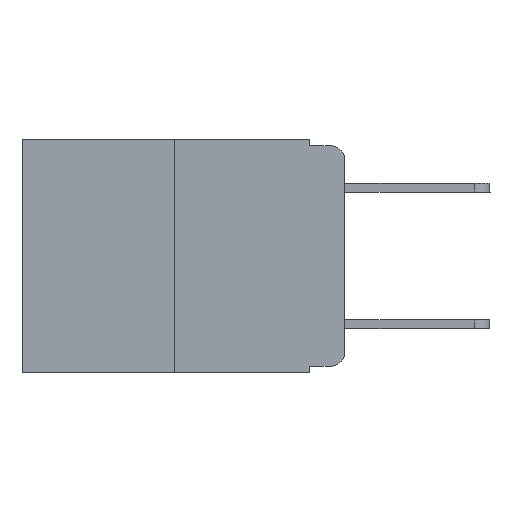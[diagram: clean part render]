
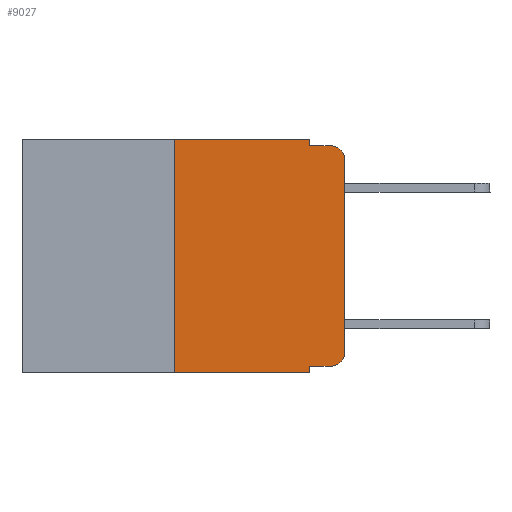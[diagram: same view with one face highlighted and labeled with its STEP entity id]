
A CAD part, left-side view. The second image highlights one B-rep face of the part: STEP entity #9027.
In plain terms, the highlighted planar face has unit normal (-1, 0, 0).
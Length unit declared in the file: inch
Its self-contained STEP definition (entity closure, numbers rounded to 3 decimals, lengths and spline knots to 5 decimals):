
#101 = LINE ( 'NONE', #2059, #4918 ) ;
#133 = LINE ( 'NONE', #5487, #2238 ) ;
#315 = DIRECTION ( 'NONE',  ( 0., -1., 0. ) ) ;
#328 = DIRECTION ( 'NONE',  ( 0., 0., -1. ) ) ;
#723 = CARTESIAN_POINT ( 'NONE',  ( 0., 0.051, -0.01 ) ) ;
#773 = CIRCLE ( 'NONE', #4574, 0.02 ) ;
#930 = ORIENTED_EDGE ( 'NONE', *, *, #2536, .F. ) ;
#1069 = AXIS2_PLACEMENT_3D ( 'NONE', #9760, #3588, #4391 ) ;
#1071 = EDGE_CURVE ( 'NONE', #6684, #6818, #6319, .T. ) ;
#1081 = CARTESIAN_POINT ( 'NONE',  ( 0., 0.473, 0. ) ) ;
#1154 = LINE ( 'NONE', #7395, #5694 ) ;
#1967 = DIRECTION ( 'NONE',  ( 0., 0., -1. ) ) ;
#2000 = EDGE_CURVE ( 'NONE', #10084, #7361, #8566, .T. ) ;
#2059 = CARTESIAN_POINT ( 'NONE',  ( 0., 0.051, 0. ) ) ;
#2163 = DIRECTION ( 'NONE',  ( -1., 0., 0. ) ) ;
#2238 = VECTOR ( 'NONE', #3946, 39.37008 ) ;
#2375 = CARTESIAN_POINT ( 'NONE',  ( 0., 0.051, -0.01 ) ) ;
#2395 = ORIENTED_EDGE ( 'NONE', *, *, #4846, .T. ) ;
#2536 = EDGE_CURVE ( 'NONE', #4348, #4883, #101, .T. ) ;
#2615 = AXIS2_PLACEMENT_3D ( 'NONE', #8414, #2163, #4628 ) ;
#2802 = DIRECTION ( 'NONE',  ( 0., -1., 0. ) ) ;
#2839 = CARTESIAN_POINT ( 'NONE',  ( 0., 0.051, -0.343 ) ) ;
#2976 = ORIENTED_EDGE ( 'NONE', *, *, #8283, .T. ) ;
#3493 = ORIENTED_EDGE ( 'NONE', *, *, #5857, .F. ) ;
#3586 = DIRECTION ( 'NONE',  ( 0., 0., 1. ) ) ;
#3588 = DIRECTION ( 'NONE',  ( 1., 0., 0. ) ) ;
#3708 = EDGE_CURVE ( 'NONE', #4954, #10084, #6498, .T. ) ;
#3941 = LINE ( 'NONE', #4165, #5410 ) ;
#3946 = DIRECTION ( 'NONE',  ( 0., 0., -1. ) ) ;
#4165 = CARTESIAN_POINT ( 'NONE',  ( 0., 0.051, -0.333 ) ) ;
#4207 = CARTESIAN_POINT ( 'NONE',  ( 0., 0.02, -0.333 ) ) ;
#4348 = VERTEX_POINT ( 'NONE', #9409 ) ;
#4374 = EDGE_CURVE ( 'NONE', #10076, #6104, #7677, .T. ) ;
#4391 = DIRECTION ( 'NONE',  ( 0., 0., -1. ) ) ;
#4407 = CARTESIAN_POINT ( 'NONE',  ( 0., 0.02, -0.313 ) ) ;
#4574 = AXIS2_PLACEMENT_3D ( 'NONE', #4407, #5123, #1967 ) ;
#4628 = DIRECTION ( 'NONE',  ( 0., 0., -1. ) ) ;
#4703 = CARTESIAN_POINT ( 'NONE',  ( 0., 0., 0. ) ) ;
#4775 = ORIENTED_EDGE ( 'NONE', *, *, #2000, .F. ) ;
#4846 = EDGE_CURVE ( 'NONE', #4954, #4883, #1154, .T. ) ;
#4883 = VERTEX_POINT ( 'NONE', #2839 ) ;
#4918 = VECTOR ( 'NONE', #328, 39.37008 ) ;
#4954 = VERTEX_POINT ( 'NONE', #8898 ) ;
#5003 = ORIENTED_EDGE ( 'NONE', *, *, #6383, .T. ) ;
#5123 = DIRECTION ( 'NONE',  ( -1., 0., 0. ) ) ;
#5276 = FACE_OUTER_BOUND ( 'NONE', #6933, .T. ) ;
#5410 = VECTOR ( 'NONE', #6280, 39.37008 ) ;
#5487 = CARTESIAN_POINT ( 'NONE',  ( 0., 0.051, 0. ) ) ;
#5499 = EDGE_CURVE ( 'NONE', #7713, #6684, #773, .T. ) ;
#5694 = VECTOR ( 'NONE', #2802, 39.37008 ) ;
#5857 = EDGE_CURVE ( 'NONE', #7361, #10076, #133, .T. ) ;
#6104 = VERTEX_POINT ( 'NONE', #9462 ) ;
#6280 = DIRECTION ( 'NONE',  ( 0., -1., 0. ) ) ;
#6319 = LINE ( 'NONE', #4703, #8135 ) ;
#6349 = DIRECTION ( 'NONE',  ( 0., -1., 0. ) ) ;
#6383 = EDGE_CURVE ( 'NONE', #6818, #6104, #9322, .T. ) ;
#6498 = LINE ( 'NONE', #7581, #7220 ) ;
#6684 = VERTEX_POINT ( 'NONE', #8740 ) ;
#6818 = VERTEX_POINT ( 'NONE', #8974 ) ;
#6933 = EDGE_LOOP ( 'NONE', ( #8978, #5003, #8326, #3493, #4775, #8273, #2395, #930, #2976, #9529 ) ) ;
#7220 = VECTOR ( 'NONE', #3586, 39.37008 ) ;
#7361 = VERTEX_POINT ( 'NONE', #8048 ) ;
#7395 = CARTESIAN_POINT ( 'NONE',  ( 0., 0.473, -0.343 ) ) ;
#7581 = CARTESIAN_POINT ( 'NONE',  ( 0., 0.25, 0. ) ) ;
#7677 = LINE ( 'NONE', #723, #8895 ) ;
#7713 = VERTEX_POINT ( 'NONE', #4207 ) ;
#8048 = CARTESIAN_POINT ( 'NONE',  ( 0., 0.051, 0. ) ) ;
#8135 = VECTOR ( 'NONE', #10170, 39.37008 ) ;
#8273 = ORIENTED_EDGE ( 'NONE', *, *, #3708, .F. ) ;
#8283 = EDGE_CURVE ( 'NONE', #4348, #7713, #3941, .T. ) ;
#8326 = ORIENTED_EDGE ( 'NONE', *, *, #4374, .F. ) ;
#8414 = CARTESIAN_POINT ( 'NONE',  ( 0., 0.02, -0.03 ) ) ;
#8566 = LINE ( 'NONE', #1081, #10172 ) ;
#8719 = CARTESIAN_POINT ( 'NONE',  ( 0., 0.25, 0. ) ) ;
#8740 = CARTESIAN_POINT ( 'NONE',  ( 0., 0., -0.313 ) ) ;
#8895 = VECTOR ( 'NONE', #6349, 39.37008 ) ;
#8898 = CARTESIAN_POINT ( 'NONE',  ( 0., 0.25, -0.343 ) ) ;
#8974 = CARTESIAN_POINT ( 'NONE',  ( 0., 0., -0.03 ) ) ;
#8975 = PLANE ( 'NONE',  #1069 ) ;
#8978 = ORIENTED_EDGE ( 'NONE', *, *, #1071, .T. ) ;
#9027 = ADVANCED_FACE ( 'NONE', ( #5276 ), #8975, .F. ) ;
#9322 = CIRCLE ( 'NONE', #2615, 0.02 ) ;
#9409 = CARTESIAN_POINT ( 'NONE',  ( 0., 0.051, -0.333 ) ) ;
#9462 = CARTESIAN_POINT ( 'NONE',  ( 0., 0.02, -0.01 ) ) ;
#9529 = ORIENTED_EDGE ( 'NONE', *, *, #5499, .T. ) ;
#9760 = CARTESIAN_POINT ( 'NONE',  ( 0., 0.473, 0. ) ) ;
#10076 = VERTEX_POINT ( 'NONE', #2375 ) ;
#10084 = VERTEX_POINT ( 'NONE', #8719 ) ;
#10170 = DIRECTION ( 'NONE',  ( 0., 0., 1. ) ) ;
#10172 = VECTOR ( 'NONE', #315, 39.37008 ) ;
